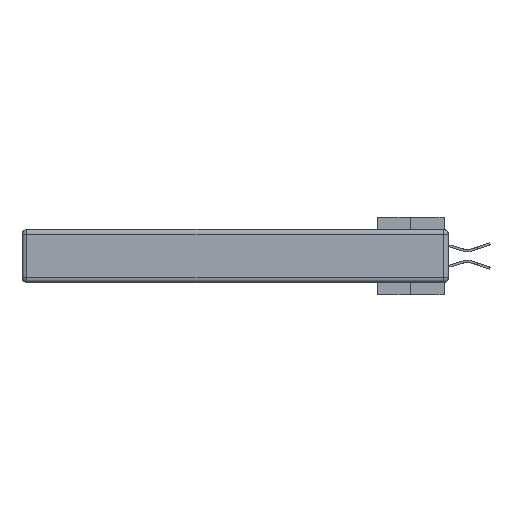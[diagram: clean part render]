
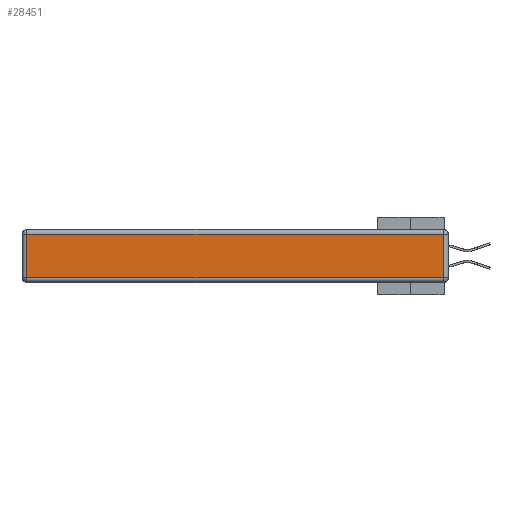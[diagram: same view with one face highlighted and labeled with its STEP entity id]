
A CAD part, left-side view. The second image highlights one B-rep face of the part: STEP entity #28451.
In plain terms, the highlighted planar face has unit normal (-1, 0, 0).
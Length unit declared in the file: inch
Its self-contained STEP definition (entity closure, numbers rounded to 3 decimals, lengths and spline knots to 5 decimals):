
#408 = PLANE ( 'NONE',  #11011 ) ;
#2302 = VECTOR ( 'NONE', #6858, 39.37008 ) ;
#3779 = CARTESIAN_POINT ( 'NONE',  ( 0., 2.72, -0.313 ) ) ;
#6858 = DIRECTION ( 'NONE',  ( 0., 1., 0. ) ) ;
#7597 = DIRECTION ( 'NONE',  ( 0., 0., -1. ) ) ;
#8345 = CARTESIAN_POINT ( 'NONE',  ( 0., 0., -0.343 ) ) ;
#10349 = EDGE_CURVE ( 'NONE', #31528, #38644, #30960, .T. ) ;
#10842 = VERTEX_POINT ( 'NONE', #20617 ) ;
#11011 = AXIS2_PLACEMENT_3D ( 'NONE', #8345, #32680, #11868 ) ;
#11515 = DIRECTION ( 'NONE',  ( 0., 0., 1. ) ) ;
#11605 = EDGE_CURVE ( 'NONE', #38644, #42693, #43863, .T. ) ;
#11868 = DIRECTION ( 'NONE',  ( 0., 0., 1. ) ) ;
#12051 = ORIENTED_EDGE ( 'NONE', *, *, #10349, .T. ) ;
#12115 = LINE ( 'NONE', #17644, #31681 ) ;
#14010 = EDGE_LOOP ( 'NONE', ( #12051, #14843, #28277, #30681 ) ) ;
#14843 = ORIENTED_EDGE ( 'NONE', *, *, #11605, .T. ) ;
#16917 = CARTESIAN_POINT ( 'NONE',  ( 0., 0.03, -0.313 ) ) ;
#17644 = CARTESIAN_POINT ( 'NONE',  ( 0., 2.72, -0.343 ) ) ;
#20268 = CARTESIAN_POINT ( 'NONE',  ( 0., 0., -0.313 ) ) ;
#20617 = CARTESIAN_POINT ( 'NONE',  ( 0., 2.72, -0.03 ) ) ;
#25096 = FACE_OUTER_BOUND ( 'NONE', #14010, .T. ) ;
#25955 = EDGE_CURVE ( 'NONE', #42693, #10842, #32245, .T. ) ;
#27030 = VECTOR ( 'NONE', #11515, 39.37008 ) ;
#28277 = ORIENTED_EDGE ( 'NONE', *, *, #25955, .T. ) ;
#28451 = ADVANCED_FACE ( 'NONE', ( #25096 ), #408, .T. ) ;
#28529 = CARTESIAN_POINT ( 'NONE',  ( 0., 0.03, -0.343 ) ) ;
#30681 = ORIENTED_EDGE ( 'NONE', *, *, #38347, .T. ) ;
#30960 = LINE ( 'NONE', #20268, #36918 ) ;
#31528 = VERTEX_POINT ( 'NONE', #3779 ) ;
#31681 = VECTOR ( 'NONE', #7597, 39.37008 ) ;
#32245 = LINE ( 'NONE', #34486, #2302 ) ;
#32680 = DIRECTION ( 'NONE',  ( -1., 0., 0. ) ) ;
#34486 = CARTESIAN_POINT ( 'NONE',  ( 0., 2.75, -0.03 ) ) ;
#36918 = VECTOR ( 'NONE', #37720, 39.37008 ) ;
#37388 = CARTESIAN_POINT ( 'NONE',  ( 0., 0.03, -0.03 ) ) ;
#37720 = DIRECTION ( 'NONE',  ( 0., -1., 0. ) ) ;
#38347 = EDGE_CURVE ( 'NONE', #10842, #31528, #12115, .T. ) ;
#38644 = VERTEX_POINT ( 'NONE', #16917 ) ;
#42693 = VERTEX_POINT ( 'NONE', #37388 ) ;
#43863 = LINE ( 'NONE', #28529, #27030 ) ;
